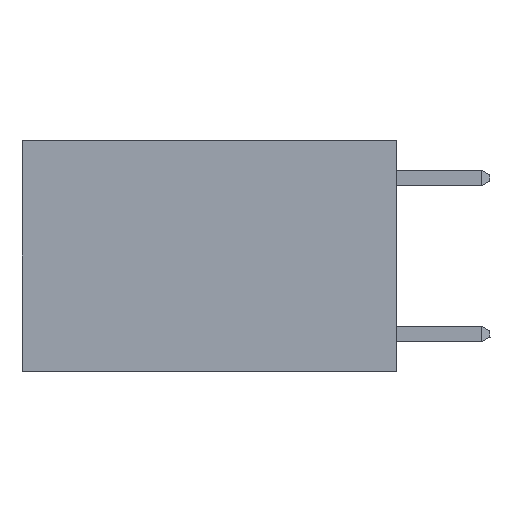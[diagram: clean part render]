
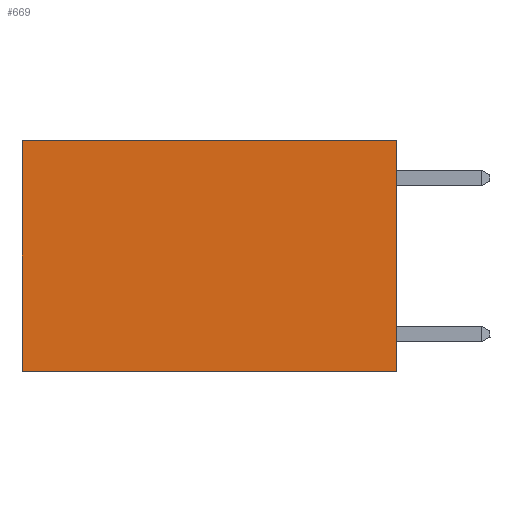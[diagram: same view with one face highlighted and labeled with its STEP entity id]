
A CAD part, left-side view. The second image highlights one B-rep face of the part: STEP entity #669.
In plain terms, the highlighted planar face has unit normal (-1, 0, 0).
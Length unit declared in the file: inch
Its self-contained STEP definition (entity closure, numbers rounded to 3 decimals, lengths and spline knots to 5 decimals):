
#170 = LINE ( 'NONE', #4428, #8579 ) ;
#172 = LINE ( 'NONE', #4410, #6281 ) ;
#258 = AXIS2_PLACEMENT_3D ( 'NONE', #1676, #1334, #1312 ) ;
#491 = ORIENTED_EDGE ( 'NONE', *, *, #2463, .F. ) ;
#669 = ADVANCED_FACE ( 'NONE', ( #10220 ), #2206, .F. ) ;
#834 = EDGE_CURVE ( 'NONE', #2941, #9034, #172, .T. ) ;
#1312 = DIRECTION ( 'NONE',  ( 0., 0., -1. ) ) ;
#1334 = DIRECTION ( 'NONE',  ( 1., 0., 0. ) ) ;
#1637 = DIRECTION ( 'NONE',  ( 0., 1., 0. ) ) ;
#1676 = CARTESIAN_POINT ( 'NONE',  ( 0.2625, 0., 0. ) ) ;
#1677 = CARTESIAN_POINT ( 'NONE',  ( 0.2625, 0., 0. ) ) ;
#2056 = DIRECTION ( 'NONE',  ( 0., 0., -1. ) ) ;
#2206 = PLANE ( 'NONE',  #258 ) ;
#2463 = EDGE_CURVE ( 'NONE', #2941, #9786, #3693, .T. ) ;
#2860 = VERTEX_POINT ( 'NONE', #9293 ) ;
#2941 = VERTEX_POINT ( 'NONE', #5489 ) ;
#3040 = VECTOR ( 'NONE', #4478, 39.37008 ) ;
#3282 = CARTESIAN_POINT ( 'NONE',  ( 0.2625, 0.6, 0. ) ) ;
#3297 = CARTESIAN_POINT ( 'NONE',  ( 0.2625, 0., -0.37 ) ) ;
#3445 = ORIENTED_EDGE ( 'NONE', *, *, #834, .T. ) ;
#3693 = LINE ( 'NONE', #1677, #4197 ) ;
#3977 = EDGE_CURVE ( 'NONE', #9034, #2860, #5110, .T. ) ;
#4197 = VECTOR ( 'NONE', #2056, 39.37008 ) ;
#4410 = CARTESIAN_POINT ( 'NONE',  ( 0.2625, 0., 0. ) ) ;
#4428 = CARTESIAN_POINT ( 'NONE',  ( 0.2625, 0., -0.37 ) ) ;
#4478 = DIRECTION ( 'NONE',  ( 0., 0., -1. ) ) ;
#4820 = EDGE_CURVE ( 'NONE', #9786, #2860, #170, .T. ) ;
#5110 = LINE ( 'NONE', #3282, #3040 ) ;
#5489 = CARTESIAN_POINT ( 'NONE',  ( 0.2625, 0., 0. ) ) ;
#5533 = EDGE_LOOP ( 'NONE', ( #5795, #8945, #491, #3445 ) ) ;
#5763 = DIRECTION ( 'NONE',  ( 0., 1., 0. ) ) ;
#5795 = ORIENTED_EDGE ( 'NONE', *, *, #3977, .T. ) ;
#6281 = VECTOR ( 'NONE', #5763, 39.37008 ) ;
#8579 = VECTOR ( 'NONE', #1637, 39.37008 ) ;
#8945 = ORIENTED_EDGE ( 'NONE', *, *, #4820, .F. ) ;
#9034 = VERTEX_POINT ( 'NONE', #9529 ) ;
#9293 = CARTESIAN_POINT ( 'NONE',  ( 0.2625, 0.6, -0.37 ) ) ;
#9529 = CARTESIAN_POINT ( 'NONE',  ( 0.2625, 0.6, 0. ) ) ;
#9786 = VERTEX_POINT ( 'NONE', #3297 ) ;
#10220 = FACE_OUTER_BOUND ( 'NONE', #5533, .T. ) ;
